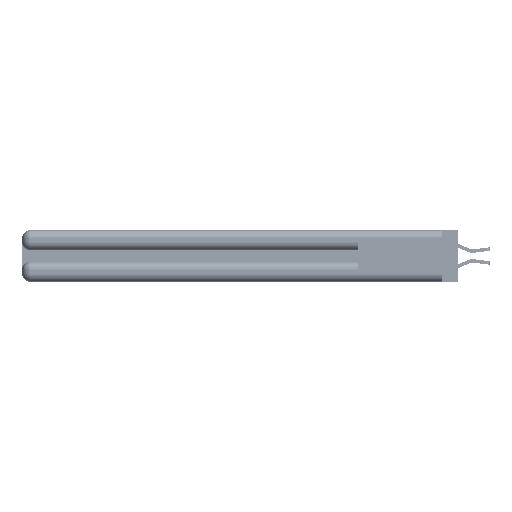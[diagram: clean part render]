
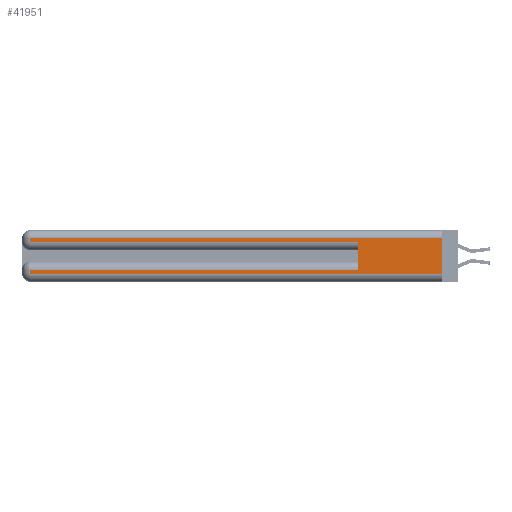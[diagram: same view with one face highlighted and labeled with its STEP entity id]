
A CAD part, left-side view. The second image highlights one B-rep face of the part: STEP entity #41951.
In plain terms, the highlighted planar face has unit normal (-1, 0, 0).
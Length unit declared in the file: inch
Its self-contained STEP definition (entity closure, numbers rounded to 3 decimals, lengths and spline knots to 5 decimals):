
#318 = ORIENTED_EDGE ( 'NONE', *, *, #12363, .F. ) ;
#2150 = VECTOR ( 'NONE', #50478, 39.37008 ) ;
#2236 = VERTEX_POINT ( 'NONE', #44891 ) ;
#2576 = LINE ( 'NONE', #31132, #24695 ) ;
#3284 = VECTOR ( 'NONE', #46312, 39.37008 ) ;
#4346 = CARTESIAN_POINT ( 'NONE',  ( 0., 2.94, 0.06 ) ) ;
#4997 = LINE ( 'NONE', #17873, #48939 ) ;
#5438 = EDGE_CURVE ( 'NONE', #2236, #15130, #2576, .T. ) ;
#5559 = CARTESIAN_POINT ( 'NONE',  ( 0., 0., 0.285 ) ) ;
#6767 = CARTESIAN_POINT ( 'NONE',  ( 0., 0., 0.06 ) ) ;
#9541 = LINE ( 'NONE', #24060, #56086 ) ;
#11332 = ORIENTED_EDGE ( 'NONE', *, *, #13862, .T. ) ;
#11891 = VECTOR ( 'NONE', #32039, 39.37008 ) ;
#11910 = CARTESIAN_POINT ( 'NONE',  ( 0., 0., 0.06 ) ) ;
#12363 = EDGE_CURVE ( 'NONE', #30153, #55352, #4997, .T. ) ;
#13363 = EDGE_CURVE ( 'NONE', #15130, #55352, #15299, .T. ) ;
#13862 = EDGE_CURVE ( 'NONE', #13898, #45924, #35352, .T. ) ;
#13898 = VERTEX_POINT ( 'NONE', #53850 ) ;
#14096 = DIRECTION ( 'NONE',  ( 1., 0., 0. ) ) ;
#15130 = VERTEX_POINT ( 'NONE', #4346 ) ;
#15299 = LINE ( 'NONE', #6767, #2150 ) ;
#16458 = VECTOR ( 'NONE', #25823, 39.37008 ) ;
#17443 = ORIENTED_EDGE ( 'NONE', *, *, #31578, .T. ) ;
#17873 = CARTESIAN_POINT ( 'NONE',  ( 0., 0., 0.37 ) ) ;
#19253 = LINE ( 'NONE', #30097, #16458 ) ;
#20075 = CARTESIAN_POINT ( 'NONE',  ( 0., 2.94, 0.37 ) ) ;
#20613 = EDGE_CURVE ( 'NONE', #30153, #54268, #19253, .T. ) ;
#21695 = VERTEX_POINT ( 'NONE', #56008 ) ;
#21759 = ORIENTED_EDGE ( 'NONE', *, *, #13363, .T. ) ;
#21834 = CARTESIAN_POINT ( 'NONE',  ( 0., 2.94, 0.31 ) ) ;
#23426 = CARTESIAN_POINT ( 'NONE',  ( 0., 0.6, 0.285 ) ) ;
#24060 = CARTESIAN_POINT ( 'NONE',  ( 0., 0.6, 0.145 ) ) ;
#24695 = VECTOR ( 'NONE', #48794, 39.37008 ) ;
#25823 = DIRECTION ( 'NONE',  ( 0., 1., 0. ) ) ;
#26754 = ORIENTED_EDGE ( 'NONE', *, *, #47772, .F. ) ;
#26988 = EDGE_LOOP ( 'NONE', ( #318, #42206, #51827, #11332, #26754, #17443, #41006, #21759 ) ) ;
#27264 = PLANE ( 'NONE',  #49936 ) ;
#28804 = LINE ( 'NONE', #38932, #50580 ) ;
#30097 = CARTESIAN_POINT ( 'NONE',  ( 0., 0., 0.31 ) ) ;
#30153 = VERTEX_POINT ( 'NONE', #34119 ) ;
#31018 = DIRECTION ( 'NONE',  ( 0., 0., -1. ) ) ;
#31132 = CARTESIAN_POINT ( 'NONE',  ( 0., 2.94, 0.37 ) ) ;
#31578 = EDGE_CURVE ( 'NONE', #21695, #2236, #28804, .T. ) ;
#31711 = CARTESIAN_POINT ( 'NONE',  ( 0., 0., 0.37 ) ) ;
#32039 = DIRECTION ( 'NONE',  ( 0., -1., 0. ) ) ;
#34119 = CARTESIAN_POINT ( 'NONE',  ( 0., 0., 0.31 ) ) ;
#35352 = LINE ( 'NONE', #5559, #11891 ) ;
#37131 = LINE ( 'NONE', #20075, #3284 ) ;
#38932 = CARTESIAN_POINT ( 'NONE',  ( 0., 0., 0.085 ) ) ;
#41006 = ORIENTED_EDGE ( 'NONE', *, *, #5438, .T. ) ;
#41951 = ADVANCED_FACE ( 'NONE', ( #47985 ), #27264, .F. ) ;
#42196 = EDGE_CURVE ( 'NONE', #54268, #13898, #37131, .T. ) ;
#42206 = ORIENTED_EDGE ( 'NONE', *, *, #20613, .T. ) ;
#43293 = DIRECTION ( 'NONE',  ( 0., 1., 0. ) ) ;
#44808 = DIRECTION ( 'NONE',  ( 0., 0., -1. ) ) ;
#44891 = CARTESIAN_POINT ( 'NONE',  ( 0., 2.94, 0.085 ) ) ;
#45924 = VERTEX_POINT ( 'NONE', #23426 ) ;
#46312 = DIRECTION ( 'NONE',  ( 0., 0., -1. ) ) ;
#47772 = EDGE_CURVE ( 'NONE', #21695, #45924, #9541, .T. ) ;
#47985 = FACE_OUTER_BOUND ( 'NONE', #26988, .T. ) ;
#48794 = DIRECTION ( 'NONE',  ( 0., 0., -1. ) ) ;
#48939 = VECTOR ( 'NONE', #31018, 39.37008 ) ;
#49936 = AXIS2_PLACEMENT_3D ( 'NONE', #31711, #14096, #44808 ) ;
#50227 = DIRECTION ( 'NONE',  ( 0., 0., 1. ) ) ;
#50478 = DIRECTION ( 'NONE',  ( 0., -1., 0. ) ) ;
#50580 = VECTOR ( 'NONE', #43293, 39.37008 ) ;
#51827 = ORIENTED_EDGE ( 'NONE', *, *, #42196, .T. ) ;
#53850 = CARTESIAN_POINT ( 'NONE',  ( 0., 2.94, 0.285 ) ) ;
#54268 = VERTEX_POINT ( 'NONE', #21834 ) ;
#55352 = VERTEX_POINT ( 'NONE', #11910 ) ;
#56008 = CARTESIAN_POINT ( 'NONE',  ( 0., 0.6, 0.085 ) ) ;
#56086 = VECTOR ( 'NONE', #50227, 39.37008 ) ;
